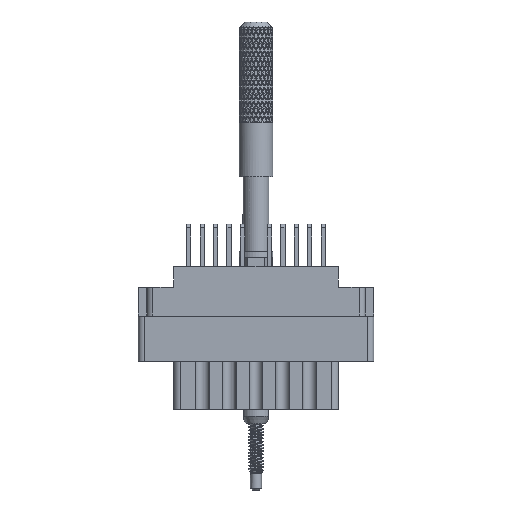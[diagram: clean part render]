
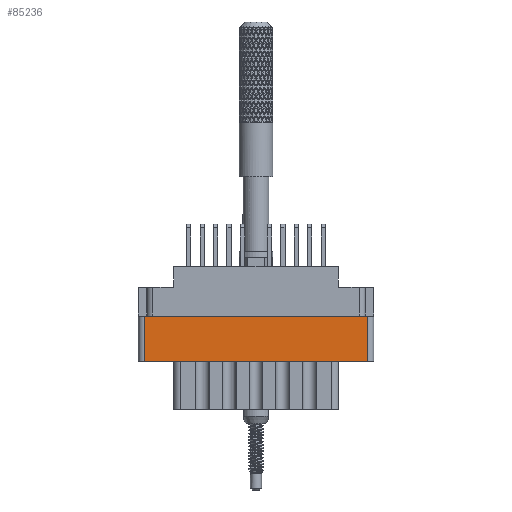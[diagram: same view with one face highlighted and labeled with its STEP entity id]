
A CAD part, front view. The second image highlights one B-rep face of the part: STEP entity #85236.
In plain terms, the highlighted planar face has unit normal (0, -1, 0).
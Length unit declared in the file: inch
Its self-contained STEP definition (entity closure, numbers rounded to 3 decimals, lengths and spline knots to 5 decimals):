
#401 = CARTESIAN_POINT ( 'NONE',  ( -0.624, -0.343, -0.277 ) ) ;
#588 = CARTESIAN_POINT ( 'NONE',  ( -0.624, -0.343, -0.798 ) ) ;
#7201 = CARTESIAN_POINT ( 'NONE',  ( 0.624, -0.343, -0.277 ) ) ;
#11146 = CARTESIAN_POINT ( 'NONE',  ( -0.656, -0.343, -0.798 ) ) ;
#14239 = VERTEX_POINT ( 'NONE', #401 ) ;
#19194 = VECTOR ( 'NONE', #56945, 39.37008 ) ;
#19754 = CARTESIAN_POINT ( 'NONE',  ( 0.624, -0.343, -0.798 ) ) ;
#28374 = EDGE_CURVE ( 'NONE', #164702, #51385, #78860, .T. ) ;
#38165 = VERTEX_POINT ( 'NONE', #98776 ) ;
#39795 = CARTESIAN_POINT ( 'NONE',  ( 0., -0.343, -0.277 ) ) ;
#43540 = EDGE_CURVE ( 'NONE', #164702, #38165, #176479, .T. ) ;
#44319 = DIRECTION ( 'NONE',  ( 0., 0., -1. ) ) ;
#44685 = ORIENTED_EDGE ( 'NONE', *, *, #28374, .T. ) ;
#46720 = ORIENTED_EDGE ( 'NONE', *, *, #77085, .F. ) ;
#51385 = VERTEX_POINT ( 'NONE', #7201 ) ;
#53030 = CARTESIAN_POINT ( 'NONE',  ( 0., -0.343, -0.529 ) ) ;
#56945 = DIRECTION ( 'NONE',  ( 1., 0., 0. ) ) ;
#58925 = ORIENTED_EDGE ( 'NONE', *, *, #43540, .F. ) ;
#61129 = EDGE_LOOP ( 'NONE', ( #46720, #117270, #58925, #44685 ) ) ;
#61720 = VECTOR ( 'NONE', #44319, 39.37008 ) ;
#63064 = VECTOR ( 'NONE', #139239, 39.37008 ) ;
#68815 = CARTESIAN_POINT ( 'NONE',  ( 0.624, -0.343, -0.529 ) ) ;
#77085 = EDGE_CURVE ( 'NONE', #14239, #51385, #125824, .T. ) ;
#78860 = LINE ( 'NONE', #19754, #142285 ) ;
#83355 = DIRECTION ( 'NONE',  ( 0., -1., 0. ) ) ;
#85236 = ADVANCED_FACE ( 'NONE', ( #145589 ), #97964, .T. ) ;
#97964 = PLANE ( 'NONE',  #182086 ) ;
#98776 = CARTESIAN_POINT ( 'NONE',  ( -0.624, -0.343, -0.529 ) ) ;
#108546 = DIRECTION ( 'NONE',  ( 0., 0., 1. ) ) ;
#117270 = ORIENTED_EDGE ( 'NONE', *, *, #133842, .T. ) ;
#122978 = LINE ( 'NONE', #588, #61720 ) ;
#125824 = LINE ( 'NONE', #39795, #19194 ) ;
#133842 = EDGE_CURVE ( 'NONE', #14239, #38165, #122978, .T. ) ;
#139239 = DIRECTION ( 'NONE',  ( -1., 0., 0. ) ) ;
#140444 = DIRECTION ( 'NONE',  ( 0., 0., -1. ) ) ;
#142285 = VECTOR ( 'NONE', #108546, 39.37008 ) ;
#145589 = FACE_OUTER_BOUND ( 'NONE', #61129, .T. ) ;
#164702 = VERTEX_POINT ( 'NONE', #68815 ) ;
#176479 = LINE ( 'NONE', #53030, #63064 ) ;
#182086 = AXIS2_PLACEMENT_3D ( 'NONE', #11146, #83355, #140444 ) ;
